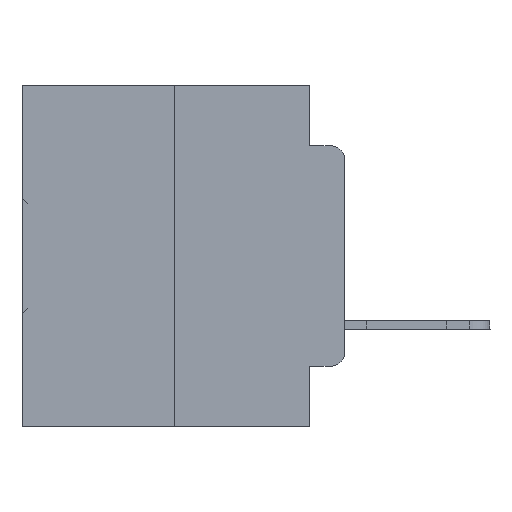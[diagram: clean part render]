
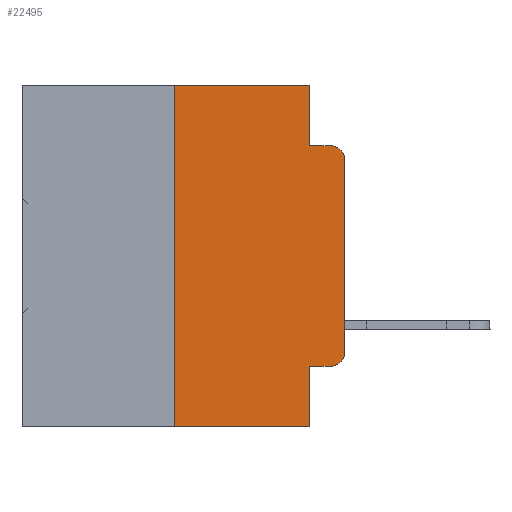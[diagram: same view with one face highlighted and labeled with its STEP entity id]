
A CAD part, left-side view. The second image highlights one B-rep face of the part: STEP entity #22495.
In plain terms, the highlighted planar face has unit normal (-1, 0, 0).
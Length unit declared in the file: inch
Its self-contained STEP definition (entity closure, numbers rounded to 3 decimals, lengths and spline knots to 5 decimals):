
#4 = VERTEX_POINT ( 'NONE', #25769 ) ;
#299 = VERTEX_POINT ( 'NONE', #2080 ) ;
#649 = AXIS2_PLACEMENT_3D ( 'NONE', #23659, #21841, #35260 ) ;
#1659 = DIRECTION ( 'NONE',  ( 0., 0., 1. ) ) ;
#2015 = EDGE_CURVE ( 'NONE', #10082, #33268, #6005, .T. ) ;
#2080 = CARTESIAN_POINT ( 'NONE',  ( 0., 0.25, 0. ) ) ;
#2455 = ORIENTED_EDGE ( 'NONE', *, *, #7065, .T. ) ;
#3131 = EDGE_CURVE ( 'NONE', #31257, #4, #14242, .T. ) ;
#3184 = VECTOR ( 'NONE', #19375, 39.37008 ) ;
#3602 = VERTEX_POINT ( 'NONE', #14331 ) ;
#4879 = LINE ( 'NONE', #26686, #8552 ) ;
#5047 = DIRECTION ( 'NONE',  ( 0., -1., 0. ) ) ;
#5826 = VECTOR ( 'NONE', #6391, 39.37008 ) ;
#6005 = CIRCLE ( 'NONE', #14000, 0.02 ) ;
#6138 = VECTOR ( 'NONE', #14489, 39.37008 ) ;
#6273 = ORIENTED_EDGE ( 'NONE', *, *, #2015, .T. ) ;
#6391 = DIRECTION ( 'NONE',  ( 0., 0., -1. ) ) ;
#6456 = CARTESIAN_POINT ( 'NONE',  ( 0., 0.051, 0. ) ) ;
#6605 = DIRECTION ( 'NONE',  ( 0., 0., 1. ) ) ;
#7065 = EDGE_CURVE ( 'NONE', #33268, #25899, #4879, .T. ) ;
#7559 = LINE ( 'NONE', #15943, #34536 ) ;
#7760 = DIRECTION ( 'NONE',  ( 1., 0., 0. ) ) ;
#8026 = ORIENTED_EDGE ( 'NONE', *, *, #20650, .F. ) ;
#8145 = CARTESIAN_POINT ( 'NONE',  ( 0., 0.473, -0.5 ) ) ;
#8479 = CARTESIAN_POINT ( 'NONE',  ( 0., 0.051, -0.4115 ) ) ;
#8552 = VECTOR ( 'NONE', #1659, 39.37008 ) ;
#9310 = LINE ( 'NONE', #33801, #6138 ) ;
#10082 = VERTEX_POINT ( 'NONE', #34250 ) ;
#10086 = DIRECTION ( 'NONE',  ( -1., 0., 0. ) ) ;
#11076 = ORIENTED_EDGE ( 'NONE', *, *, #23201, .F. ) ;
#11412 = ORIENTED_EDGE ( 'NONE', *, *, #25996, .F. ) ;
#11504 = ORIENTED_EDGE ( 'NONE', *, *, #31907, .T. ) ;
#13658 = LINE ( 'NONE', #30125, #31941 ) ;
#14000 = AXIS2_PLACEMENT_3D ( 'NONE', #23675, #10086, #31886 ) ;
#14164 = VECTOR ( 'NONE', #6605, 39.37008 ) ;
#14242 = LINE ( 'NONE', #14781, #5826 ) ;
#14331 = CARTESIAN_POINT ( 'NONE',  ( 0., 0.051, -0.4115 ) ) ;
#14489 = DIRECTION ( 'NONE',  ( 0., 0., -1. ) ) ;
#14781 = CARTESIAN_POINT ( 'NONE',  ( 0., 0.051, 0. ) ) ;
#14919 = CIRCLE ( 'NONE', #649, 0.02 ) ;
#15434 = PLANE ( 'NONE',  #22118 ) ;
#15943 = CARTESIAN_POINT ( 'NONE',  ( 0., 0.051, -0.0885 ) ) ;
#15999 = LINE ( 'NONE', #8479, #25686 ) ;
#16953 = CARTESIAN_POINT ( 'NONE',  ( 0., 0.25, 0. ) ) ;
#17034 = LINE ( 'NONE', #8145, #3184 ) ;
#17136 = ORIENTED_EDGE ( 'NONE', *, *, #26021, .T. ) ;
#18851 = DIRECTION ( 'NONE',  ( 0., -1., 0. ) ) ;
#19050 = EDGE_CURVE ( 'NONE', #4, #31913, #7559, .T. ) ;
#19375 = DIRECTION ( 'NONE',  ( 0., -1., 0. ) ) ;
#20650 = EDGE_CURVE ( 'NONE', #3602, #31750, #9310, .T. ) ;
#21026 = CARTESIAN_POINT ( 'NONE',  ( 0., 0.051, -0.5 ) ) ;
#21212 = ORIENTED_EDGE ( 'NONE', *, *, #3131, .F. ) ;
#21841 = DIRECTION ( 'NONE',  ( -1., 0., 0. ) ) ;
#22118 = AXIS2_PLACEMENT_3D ( 'NONE', #34917, #7760, #29223 ) ;
#22232 = CARTESIAN_POINT ( 'NONE',  ( 0., 0.02, -0.0885 ) ) ;
#22495 = ADVANCED_FACE ( 'NONE', ( #32238 ), #15434, .F. ) ;
#22497 = ORIENTED_EDGE ( 'NONE', *, *, #27669, .T. ) ;
#23201 = EDGE_CURVE ( 'NONE', #28187, #299, #25387, .T. ) ;
#23659 = CARTESIAN_POINT ( 'NONE',  ( 0., 0.02, -0.1085 ) ) ;
#23675 = CARTESIAN_POINT ( 'NONE',  ( 0., 0.02, -0.3915 ) ) ;
#24055 = CARTESIAN_POINT ( 'NONE',  ( 0., 0., -0.1085 ) ) ;
#25387 = LINE ( 'NONE', #16953, #14164 ) ;
#25686 = VECTOR ( 'NONE', #18851, 39.37008 ) ;
#25769 = CARTESIAN_POINT ( 'NONE',  ( 0., 0.051, -0.0885 ) ) ;
#25899 = VERTEX_POINT ( 'NONE', #24055 ) ;
#25996 = EDGE_CURVE ( 'NONE', #299, #31257, #13658, .T. ) ;
#26021 = EDGE_CURVE ( 'NONE', #3602, #10082, #15999, .T. ) ;
#26654 = CARTESIAN_POINT ( 'NONE',  ( 0., 0.25, -0.5 ) ) ;
#26686 = CARTESIAN_POINT ( 'NONE',  ( 0., 0., 0. ) ) ;
#27151 = CARTESIAN_POINT ( 'NONE',  ( 0., 0., -0.3915 ) ) ;
#27669 = EDGE_CURVE ( 'NONE', #25899, #31913, #14919, .T. ) ;
#28187 = VERTEX_POINT ( 'NONE', #26654 ) ;
#29017 = EDGE_LOOP ( 'NONE', ( #2455, #22497, #32277, #21212, #11412, #11076, #11504, #8026, #17136, #6273 ) ) ;
#29223 = DIRECTION ( 'NONE',  ( 0., 0., -1. ) ) ;
#30125 = CARTESIAN_POINT ( 'NONE',  ( 0., 0.473, 0. ) ) ;
#30289 = DIRECTION ( 'NONE',  ( 0., -1., 0. ) ) ;
#31257 = VERTEX_POINT ( 'NONE', #6456 ) ;
#31750 = VERTEX_POINT ( 'NONE', #21026 ) ;
#31886 = DIRECTION ( 'NONE',  ( 0., 0., -1. ) ) ;
#31907 = EDGE_CURVE ( 'NONE', #28187, #31750, #17034, .T. ) ;
#31913 = VERTEX_POINT ( 'NONE', #22232 ) ;
#31941 = VECTOR ( 'NONE', #30289, 39.37008 ) ;
#32238 = FACE_OUTER_BOUND ( 'NONE', #29017, .T. ) ;
#32277 = ORIENTED_EDGE ( 'NONE', *, *, #19050, .F. ) ;
#33268 = VERTEX_POINT ( 'NONE', #27151 ) ;
#33801 = CARTESIAN_POINT ( 'NONE',  ( 0., 0.051, 0. ) ) ;
#34250 = CARTESIAN_POINT ( 'NONE',  ( 0., 0.02, -0.4115 ) ) ;
#34536 = VECTOR ( 'NONE', #5047, 39.37008 ) ;
#34917 = CARTESIAN_POINT ( 'NONE',  ( 0., 0.473, 0. ) ) ;
#35260 = DIRECTION ( 'NONE',  ( 0., 0., -1. ) ) ;
